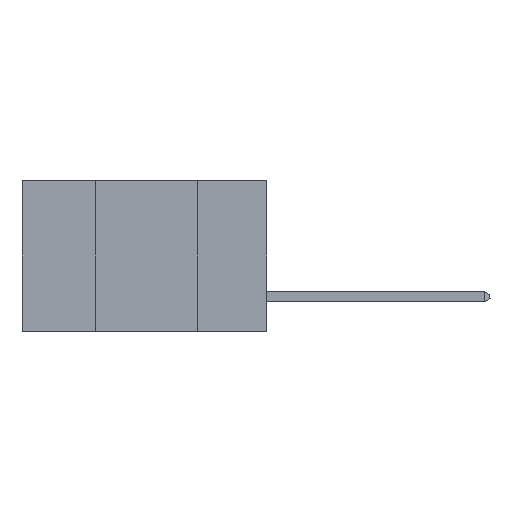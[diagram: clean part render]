
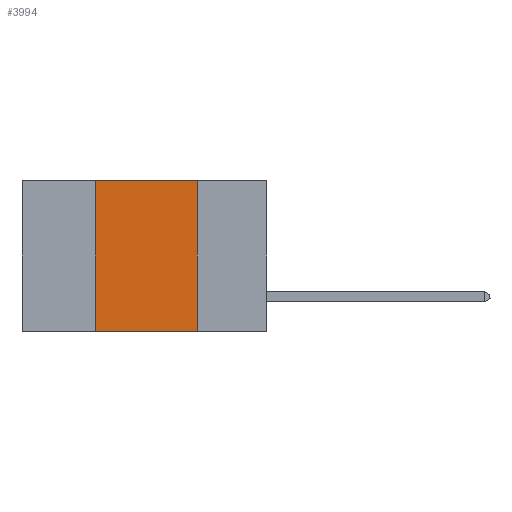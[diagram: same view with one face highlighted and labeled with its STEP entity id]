
A CAD part, left-side view. The second image highlights one B-rep face of the part: STEP entity #3994.
In plain terms, the highlighted planar face has unit normal (-1, 0, 0).
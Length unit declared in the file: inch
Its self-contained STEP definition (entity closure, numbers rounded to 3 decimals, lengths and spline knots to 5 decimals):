
#62 = DIRECTION ( 'NONE',  ( 0., -1., 0. ) ) ;
#640 = CARTESIAN_POINT ( 'NONE',  ( 0., 0.17, 0. ) ) ;
#814 = CARTESIAN_POINT ( 'NONE',  ( 0., 0.17, -0.37 ) ) ;
#1014 = ORIENTED_EDGE ( 'NONE', *, *, #5788, .F. ) ;
#1892 = ORIENTED_EDGE ( 'NONE', *, *, #11633, .F. ) ;
#2002 = EDGE_LOOP ( 'NONE', ( #1892, #1014, #14966, #5137 ) ) ;
#2146 = VERTEX_POINT ( 'NONE', #6454 ) ;
#3095 = PLANE ( 'NONE',  #4421 ) ;
#3939 = VERTEX_POINT ( 'NONE', #814 ) ;
#3981 = CARTESIAN_POINT ( 'NONE',  ( 0., 0.6, -0.37 ) ) ;
#3994 = ADVANCED_FACE ( 'NONE', ( #8476 ), #3095, .F. ) ;
#4421 = AXIS2_PLACEMENT_3D ( 'NONE', #14620, #11080, #11176 ) ;
#4795 = VECTOR ( 'NONE', #8248, 39.37008 ) ;
#4818 = CARTESIAN_POINT ( 'NONE',  ( 0., 0.42, 0. ) ) ;
#5137 = ORIENTED_EDGE ( 'NONE', *, *, #10078, .T. ) ;
#5179 = LINE ( 'NONE', #4818, #4795 ) ;
#5193 = VERTEX_POINT ( 'NONE', #8766 ) ;
#5788 = EDGE_CURVE ( 'NONE', #5193, #2146, #11696, .T. ) ;
#6022 = CARTESIAN_POINT ( 'NONE',  ( 0., 0.6, 0. ) ) ;
#6454 = CARTESIAN_POINT ( 'NONE',  ( 0., 0.17, 0. ) ) ;
#6859 = VECTOR ( 'NONE', #14425, 39.37008 ) ;
#7387 = CARTESIAN_POINT ( 'NONE',  ( 0., 0.42, -0.37 ) ) ;
#8248 = DIRECTION ( 'NONE',  ( 0., 0., 1. ) ) ;
#8476 = FACE_OUTER_BOUND ( 'NONE', #2002, .T. ) ;
#8766 = CARTESIAN_POINT ( 'NONE',  ( 0., 0.42, 0. ) ) ;
#9156 = VECTOR ( 'NONE', #13344, 39.37008 ) ;
#9950 = LINE ( 'NONE', #3981, #6859 ) ;
#10078 = EDGE_CURVE ( 'NONE', #11648, #3939, #9950, .T. ) ;
#11080 = DIRECTION ( 'NONE',  ( 1., 0., 0. ) ) ;
#11176 = DIRECTION ( 'NONE',  ( 0., 0., -1. ) ) ;
#11633 = EDGE_CURVE ( 'NONE', #2146, #3939, #14585, .T. ) ;
#11648 = VERTEX_POINT ( 'NONE', #7387 ) ;
#11696 = LINE ( 'NONE', #6022, #12780 ) ;
#12780 = VECTOR ( 'NONE', #62, 39.37008 ) ;
#13344 = DIRECTION ( 'NONE',  ( 0., 0., -1. ) ) ;
#14425 = DIRECTION ( 'NONE',  ( 0., -1., 0. ) ) ;
#14585 = LINE ( 'NONE', #640, #9156 ) ;
#14620 = CARTESIAN_POINT ( 'NONE',  ( 0., 0.6, 0. ) ) ;
#14642 = EDGE_CURVE ( 'NONE', #11648, #5193, #5179, .T. ) ;
#14966 = ORIENTED_EDGE ( 'NONE', *, *, #14642, .F. ) ;
